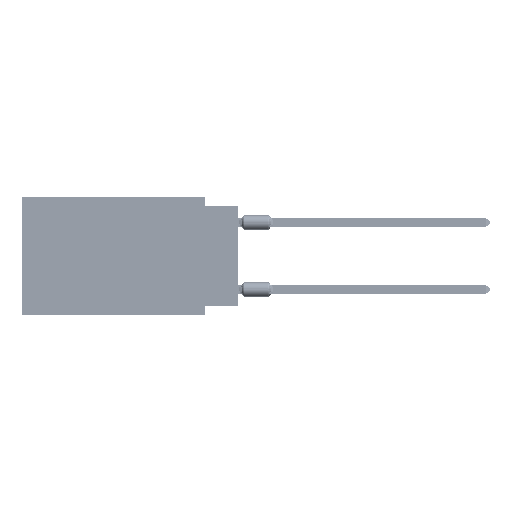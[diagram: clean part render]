
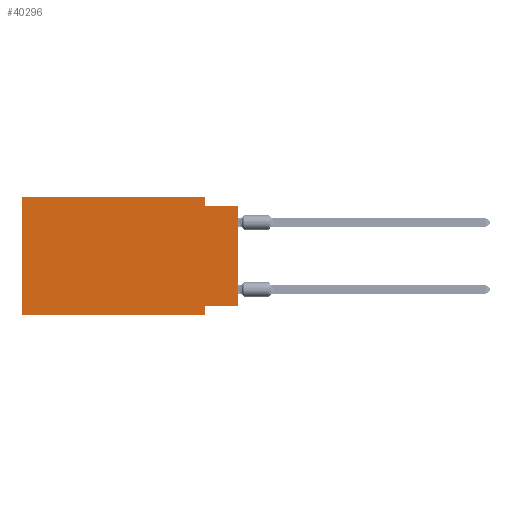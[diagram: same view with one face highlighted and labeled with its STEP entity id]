
A CAD part, left-side view. The second image highlights one B-rep face of the part: STEP entity #40296.
In plain terms, the highlighted planar face has unit normal (-1, 0, 0).
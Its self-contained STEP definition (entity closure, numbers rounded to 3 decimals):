
#667 = VERTEX_POINT ( 'NONE', #11678 ) ;
#1649 = DIRECTION ( 'NONE',  ( 0., 0., 1. ) ) ;
#2389 = VERTEX_POINT ( 'NONE', #5761 ) ;
#3029 = CARTESIAN_POINT ( 'NONE',  ( 0., 2.54, -8.89 ) ) ;
#3330 = CARTESIAN_POINT ( 'NONE',  ( 0., 16.383, -8.89 ) ) ;
#5704 = ORIENTED_EDGE ( 'NONE', *, *, #42300, .T. ) ;
#5761 = CARTESIAN_POINT ( 'NONE',  ( 0., 2.54, -8.255 ) ) ;
#5892 = DIRECTION ( 'NONE',  ( 0., 1., 0. ) ) ;
#7721 = VECTOR ( 'NONE', #46987, 1000. ) ;
#9945 = EDGE_CURVE ( 'NONE', #53395, #85274, #34869, .T. ) ;
#10238 = VECTOR ( 'NONE', #5892, 1000. ) ;
#11678 = CARTESIAN_POINT ( 'NONE',  ( 0., 16.383, 0. ) ) ;
#12651 = CARTESIAN_POINT ( 'NONE',  ( 0., 0., 0. ) ) ;
#13318 = EDGE_CURVE ( 'NONE', #43537, #66034, #54451, .T. ) ;
#14564 = CARTESIAN_POINT ( 'NONE',  ( 0., 2.54, -8.89 ) ) ;
#16271 = VECTOR ( 'NONE', #85931, 1000. ) ;
#23591 = VECTOR ( 'NONE', #64335, 1000. ) ;
#24247 = EDGE_LOOP ( 'NONE', ( #56541, #60238, #83732, #29558, #60215, #5704, #29194, #40491 ) ) ;
#24294 = LINE ( 'NONE', #3029, #7721 ) ;
#28104 = EDGE_CURVE ( 'NONE', #59245, #667, #59613, .T. ) ;
#29194 = ORIENTED_EDGE ( 'NONE', *, *, #91346, .F. ) ;
#29558 = ORIENTED_EDGE ( 'NONE', *, *, #65526, .F. ) ;
#31051 = CARTESIAN_POINT ( 'NONE',  ( 0., 2.54, -0.635 ) ) ;
#34240 = CARTESIAN_POINT ( 'NONE',  ( 0., 16.383, 0. ) ) ;
#34869 = LINE ( 'NONE', #12651, #23591 ) ;
#35844 = VECTOR ( 'NONE', #95029, 1000. ) ;
#36122 = LINE ( 'NONE', #65583, #35844 ) ;
#39084 = EDGE_CURVE ( 'NONE', #66034, #85274, #36122, .T. ) ;
#40296 = ADVANCED_FACE ( 'NONE', ( #44784 ), #48860, .F. ) ;
#40491 = ORIENTED_EDGE ( 'NONE', *, *, #85038, .F. ) ;
#41516 = VECTOR ( 'NONE', #77633, 1000. ) ;
#41608 = CARTESIAN_POINT ( 'NONE',  ( 0., 16.383, 0. ) ) ;
#41886 = CARTESIAN_POINT ( 'NONE',  ( 0., 0., -8.255 ) ) ;
#42300 = EDGE_CURVE ( 'NONE', #59245, #85067, #72166, .T. ) ;
#43158 = CARTESIAN_POINT ( 'NONE',  ( 0., 16.383, -8.89 ) ) ;
#43537 = VERTEX_POINT ( 'NONE', #83778 ) ;
#44314 = DIRECTION ( 'NONE',  ( 1., 0., 0. ) ) ;
#44784 = FACE_OUTER_BOUND ( 'NONE', #24247, .T. ) ;
#46987 = DIRECTION ( 'NONE',  ( 0., 0., -1. ) ) ;
#47212 = CARTESIAN_POINT ( 'NONE',  ( 0., 2.54, 0. ) ) ;
#47398 = VECTOR ( 'NONE', #72627, 1000. ) ;
#48860 = PLANE ( 'NONE',  #85322 ) ;
#50316 = CARTESIAN_POINT ( 'NONE',  ( 0., 0., -8.255 ) ) ;
#53395 = VERTEX_POINT ( 'NONE', #41886 ) ;
#54451 = LINE ( 'NONE', #47212, #41516 ) ;
#56541 = ORIENTED_EDGE ( 'NONE', *, *, #9945, .T. ) ;
#59245 = VERTEX_POINT ( 'NONE', #3330 ) ;
#59613 = LINE ( 'NONE', #75069, #80940 ) ;
#60215 = ORIENTED_EDGE ( 'NONE', *, *, #28104, .F. ) ;
#60238 = ORIENTED_EDGE ( 'NONE', *, *, #39084, .F. ) ;
#61835 = CARTESIAN_POINT ( 'NONE',  ( 0., 0., -0.635 ) ) ;
#63834 = DIRECTION ( 'NONE',  ( 0., 0., -1. ) ) ;
#64335 = DIRECTION ( 'NONE',  ( 0., 0., 1. ) ) ;
#65526 = EDGE_CURVE ( 'NONE', #667, #43537, #71432, .T. ) ;
#65583 = CARTESIAN_POINT ( 'NONE',  ( 0., 0., -0.635 ) ) ;
#66034 = VERTEX_POINT ( 'NONE', #31051 ) ;
#71432 = LINE ( 'NONE', #34240, #16271 ) ;
#72166 = LINE ( 'NONE', #43158, #47398 ) ;
#72627 = DIRECTION ( 'NONE',  ( 0., -1., 0. ) ) ;
#75069 = CARTESIAN_POINT ( 'NONE',  ( 0., 16.383, 0. ) ) ;
#77633 = DIRECTION ( 'NONE',  ( 0., 0., -1. ) ) ;
#80940 = VECTOR ( 'NONE', #1649, 1000. ) ;
#83732 = ORIENTED_EDGE ( 'NONE', *, *, #13318, .F. ) ;
#83778 = CARTESIAN_POINT ( 'NONE',  ( 0., 2.54, 0. ) ) ;
#85038 = EDGE_CURVE ( 'NONE', #53395, #2389, #87977, .T. ) ;
#85067 = VERTEX_POINT ( 'NONE', #14564 ) ;
#85274 = VERTEX_POINT ( 'NONE', #61835 ) ;
#85322 = AXIS2_PLACEMENT_3D ( 'NONE', #41608, #44314, #63834 ) ;
#85931 = DIRECTION ( 'NONE',  ( 0., -1., 0. ) ) ;
#87977 = LINE ( 'NONE', #50316, #10238 ) ;
#91346 = EDGE_CURVE ( 'NONE', #2389, #85067, #24294, .T. ) ;
#95029 = DIRECTION ( 'NONE',  ( 0., -1., 0. ) ) ;
